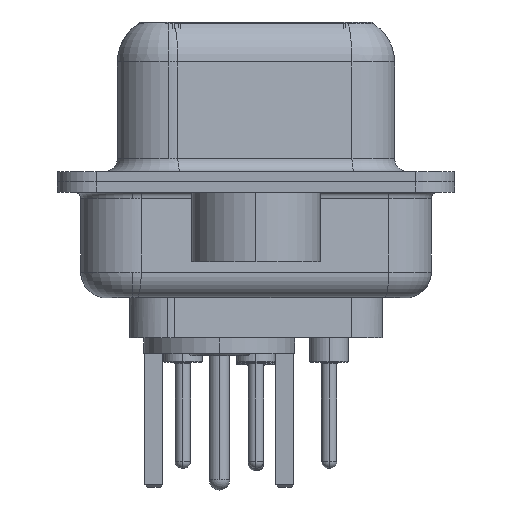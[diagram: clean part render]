
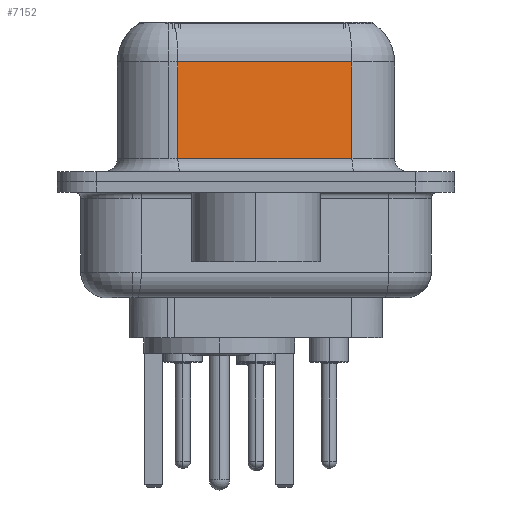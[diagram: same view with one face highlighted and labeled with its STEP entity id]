
A CAD part, left-side view. The second image highlights one B-rep face of the part: STEP entity #7152.
In plain terms, the highlighted planar face has unit normal (-0.985, -0.174, 0).
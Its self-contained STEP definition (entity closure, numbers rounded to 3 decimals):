
#324 = VECTOR ( 'NONE', #17018, 1000. ) ;
#1401 = CARTESIAN_POINT ( 'NONE',  ( 4.43, 3.028, 4.65 ) ) ;
#3168 = ORIENTED_EDGE ( 'NONE', *, *, #31100, .F. ) ;
#7152 = ADVANCED_FACE ( 'NONE', ( #23718 ), #34298, .F. ) ;
#7465 = LINE ( 'NONE', #7682, #18706 ) ;
#7682 = CARTESIAN_POINT ( 'NONE',  ( 5.621, -3.722, 4.65 ) ) ;
#8299 = VERTEX_POINT ( 'NONE', #1401 ) ;
#9321 = EDGE_CURVE ( 'NONE', #13582, #29539, #15849, .T. ) ;
#10100 = DIRECTION ( 'NONE',  ( -0.174, 0.985, 0. ) ) ;
#11197 = VECTOR ( 'NONE', #35041, 1000. ) ;
#11479 = EDGE_CURVE ( 'NONE', #14239, #8299, #7465, .T. ) ;
#13582 = VERTEX_POINT ( 'NONE', #25031 ) ;
#14044 = VECTOR ( 'NONE', #27110, 1000. ) ;
#14239 = VERTEX_POINT ( 'NONE', #22561 ) ;
#14571 = CARTESIAN_POINT ( 'NONE',  ( 5.621, -3.722, 0.9 ) ) ;
#15779 = CARTESIAN_POINT ( 'NONE',  ( 5.621, -3.722, 0.9 ) ) ;
#15849 = LINE ( 'NONE', #14571, #324 ) ;
#17018 = DIRECTION ( 'NONE',  ( 0.174, -0.985, 0. ) ) ;
#17222 = EDGE_CURVE ( 'NONE', #8299, #13582, #30852, .T. ) ;
#18281 = DIRECTION ( 'NONE',  ( 0.985, 0.174, 0. ) ) ;
#18706 = VECTOR ( 'NONE', #10100, 1000. ) ;
#21229 = EDGE_LOOP ( 'NONE', ( #3168, #33135, #31206, #29205 ) ) ;
#22561 = CARTESIAN_POINT ( 'NONE',  ( 5.621, -3.722, 4.65 ) ) ;
#23718 = FACE_OUTER_BOUND ( 'NONE', #21229, .T. ) ;
#24349 = CARTESIAN_POINT ( 'NONE',  ( 4.43, 3.028, 6.4 ) ) ;
#25031 = CARTESIAN_POINT ( 'NONE',  ( 4.43, 3.028, 0.9 ) ) ;
#25947 = AXIS2_PLACEMENT_3D ( 'NONE', #34537, #18281, #26103 ) ;
#26103 = DIRECTION ( 'NONE',  ( -0.174, 0.985, 0. ) ) ;
#27110 = DIRECTION ( 'NONE',  ( 0., 0., -1. ) ) ;
#29205 = ORIENTED_EDGE ( 'NONE', *, *, #9321, .T. ) ;
#29539 = VERTEX_POINT ( 'NONE', #15779 ) ;
#30852 = LINE ( 'NONE', #24349, #14044 ) ;
#31100 = EDGE_CURVE ( 'NONE', #14239, #29539, #32311, .T. ) ;
#31206 = ORIENTED_EDGE ( 'NONE', *, *, #17222, .T. ) ;
#32177 = CARTESIAN_POINT ( 'NONE',  ( 5.621, -3.722, 6.4 ) ) ;
#32311 = LINE ( 'NONE', #32177, #11197 ) ;
#33135 = ORIENTED_EDGE ( 'NONE', *, *, #11479, .T. ) ;
#34298 = PLANE ( 'NONE',  #25947 ) ;
#34537 = CARTESIAN_POINT ( 'NONE',  ( 5.621, -3.722, 6.4 ) ) ;
#35041 = DIRECTION ( 'NONE',  ( 0., 0., -1. ) ) ;
